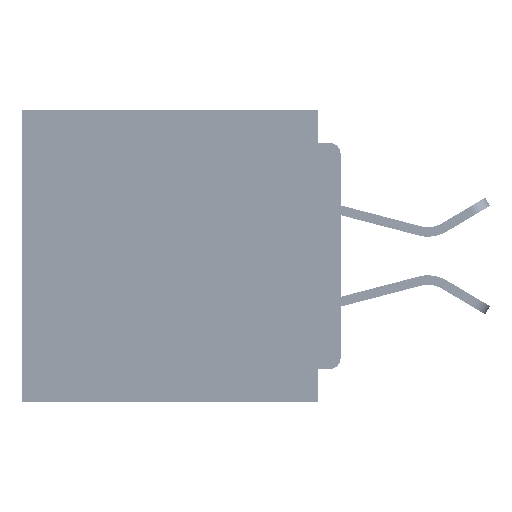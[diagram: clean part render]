
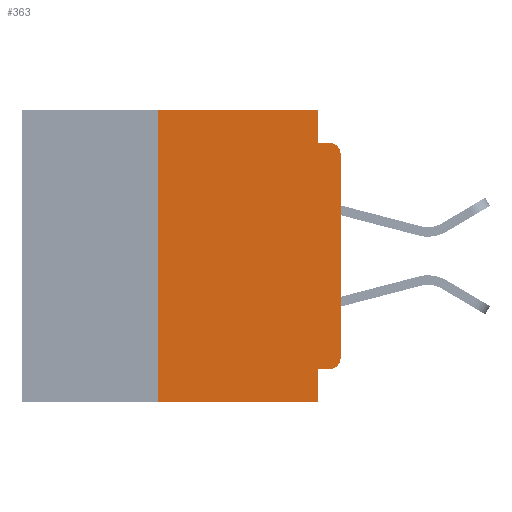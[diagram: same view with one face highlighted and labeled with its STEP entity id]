
A CAD part, left-side view. The second image highlights one B-rep face of the part: STEP entity #363.
In plain terms, the highlighted planar face has unit normal (-1, 0, 0).
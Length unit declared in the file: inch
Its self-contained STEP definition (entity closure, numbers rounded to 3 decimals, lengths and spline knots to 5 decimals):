
#234 = CARTESIAN_POINT ( 'NONE',  ( 0., 0.031, -0.045 ) ) ;
#363 = ADVANCED_FACE ( 'NONE', ( #35734 ), #36285, .F. ) ;
#1789 = DIRECTION ( 'NONE',  ( 0., 0., -1. ) ) ;
#2065 = AXIS2_PLACEMENT_3D ( 'NONE', #30913, #5976, #35728 ) ;
#2545 = EDGE_CURVE ( 'NONE', #19469, #3942, #49190, .T. ) ;
#3942 = VERTEX_POINT ( 'NONE', #12374 ) ;
#4067 = CARTESIAN_POINT ( 'NONE',  ( 0., 0.437, 0. ) ) ;
#4330 = ORIENTED_EDGE ( 'NONE', *, *, #42523, .T. ) ;
#4727 = CARTESIAN_POINT ( 'NONE',  ( 0., 0.031, -0.4 ) ) ;
#5724 = LINE ( 'NONE', #27153, #24837 ) ;
#5976 = DIRECTION ( 'NONE',  ( 1., 0., 0. ) ) ;
#6121 = LINE ( 'NONE', #38951, #37306 ) ;
#6165 = VECTOR ( 'NONE', #39838, 39.37008 ) ;
#6410 = ORIENTED_EDGE ( 'NONE', *, *, #41505, .T. ) ;
#7679 = LINE ( 'NONE', #4067, #26753 ) ;
#9474 = CARTESIAN_POINT ( 'NONE',  ( 0., 0.015, -0.045 ) ) ;
#10599 = LINE ( 'NONE', #19923, #30962 ) ;
#10759 = ORIENTED_EDGE ( 'NONE', *, *, #28411, .F. ) ;
#11155 = DIRECTION ( 'NONE',  ( 0., 0., 1. ) ) ;
#11517 = ORIENTED_EDGE ( 'NONE', *, *, #39396, .T. ) ;
#11683 = CARTESIAN_POINT ( 'NONE',  ( 0., 0.25, -0.4 ) ) ;
#11711 = EDGE_LOOP ( 'NONE', ( #11517, #6410, #13420, #52088, #10759, #29850, #4330, #13935, #52042, #15812 ) ) ;
#11923 = CARTESIAN_POINT ( 'NONE',  ( 0., 0.25, -0.4 ) ) ;
#12323 = EDGE_CURVE ( 'NONE', #33633, #23144, #5724, .T. ) ;
#12374 = CARTESIAN_POINT ( 'NONE',  ( 0., 0.25, 0. ) ) ;
#12680 = VERTEX_POINT ( 'NONE', #37437 ) ;
#12895 = VERTEX_POINT ( 'NONE', #23193 ) ;
#13278 = CARTESIAN_POINT ( 'NONE',  ( 0., 0.031, -0.355 ) ) ;
#13420 = ORIENTED_EDGE ( 'NONE', *, *, #12323, .F. ) ;
#13935 = ORIENTED_EDGE ( 'NONE', *, *, #35144, .F. ) ;
#13942 = CIRCLE ( 'NONE', #32953, 0.015 ) ;
#14894 = DIRECTION ( 'NONE',  ( 0., -1., 0. ) ) ;
#15812 = ORIENTED_EDGE ( 'NONE', *, *, #35626, .T. ) ;
#16298 = CARTESIAN_POINT ( 'NONE',  ( 0., 0., 0. ) ) ;
#16793 = VECTOR ( 'NONE', #11155, 39.37008 ) ;
#17746 = CARTESIAN_POINT ( 'NONE',  ( 0., 0.015, -0.34 ) ) ;
#18173 = EDGE_CURVE ( 'NONE', #12680, #33633, #27457, .T. ) ;
#18257 = LINE ( 'NONE', #35788, #6165 ) ;
#19469 = VERTEX_POINT ( 'NONE', #11923 ) ;
#19923 = CARTESIAN_POINT ( 'NONE',  ( 0., 0., -0.355 ) ) ;
#20084 = VERTEX_POINT ( 'NONE', #4727 ) ;
#20437 = VECTOR ( 'NONE', #48788, 39.37008 ) ;
#21707 = LINE ( 'NONE', #16298, #20437 ) ;
#21852 = DIRECTION ( 'NONE',  ( 0., 0., -1. ) ) ;
#23144 = VERTEX_POINT ( 'NONE', #9474 ) ;
#23193 = CARTESIAN_POINT ( 'NONE',  ( 0., 0., -0.06 ) ) ;
#23903 = CIRCLE ( 'NONE', #32817, 0.015 ) ;
#24019 = DIRECTION ( 'NONE',  ( 0., 1., 0. ) ) ;
#24179 = VERTEX_POINT ( 'NONE', #24302 ) ;
#24302 = CARTESIAN_POINT ( 'NONE',  ( 0., 0.015, -0.355 ) ) ;
#24837 = VECTOR ( 'NONE', #14894, 39.37008 ) ;
#24910 = VECTOR ( 'NONE', #43982, 39.37008 ) ;
#25299 = VERTEX_POINT ( 'NONE', #13278 ) ;
#26234 = DIRECTION ( 'NONE',  ( -1., 0., 0. ) ) ;
#26714 = DIRECTION ( 'NONE',  ( 0., 0., -1. ) ) ;
#26753 = VECTOR ( 'NONE', #48884, 39.37008 ) ;
#27153 = CARTESIAN_POINT ( 'NONE',  ( 0., 0., -0.045 ) ) ;
#27457 = LINE ( 'NONE', #27649, #24910 ) ;
#27649 = CARTESIAN_POINT ( 'NONE',  ( 0., 0.031, 0. ) ) ;
#28411 = EDGE_CURVE ( 'NONE', #3942, #12680, #7679, .T. ) ;
#29850 = ORIENTED_EDGE ( 'NONE', *, *, #2545, .F. ) ;
#30913 = CARTESIAN_POINT ( 'NONE',  ( 0., 0.437, 0. ) ) ;
#30962 = VECTOR ( 'NONE', #24019, 39.37008 ) ;
#32817 = AXIS2_PLACEMENT_3D ( 'NONE', #17746, #46175, #21852 ) ;
#32953 = AXIS2_PLACEMENT_3D ( 'NONE', #50543, #26234, #1789 ) ;
#33633 = VERTEX_POINT ( 'NONE', #234 ) ;
#35144 = EDGE_CURVE ( 'NONE', #25299, #20084, #6121, .T. ) ;
#35626 = EDGE_CURVE ( 'NONE', #24179, #52208, #23903, .T. ) ;
#35728 = DIRECTION ( 'NONE',  ( 0., 0., -1. ) ) ;
#35734 = FACE_OUTER_BOUND ( 'NONE', #11711, .T. ) ;
#35788 = CARTESIAN_POINT ( 'NONE',  ( 0., 0.437, -0.4 ) ) ;
#36285 = PLANE ( 'NONE',  #2065 ) ;
#37306 = VECTOR ( 'NONE', #26714, 39.37008 ) ;
#37437 = CARTESIAN_POINT ( 'NONE',  ( 0., 0.031, 0. ) ) ;
#38951 = CARTESIAN_POINT ( 'NONE',  ( 0., 0.031, -0.4 ) ) ;
#39396 = EDGE_CURVE ( 'NONE', #52208, #12895, #21707, .T. ) ;
#39838 = DIRECTION ( 'NONE',  ( 0., -1., 0. ) ) ;
#41505 = EDGE_CURVE ( 'NONE', #12895, #23144, #13942, .T. ) ;
#42523 = EDGE_CURVE ( 'NONE', #19469, #20084, #18257, .T. ) ;
#43123 = CARTESIAN_POINT ( 'NONE',  ( 0., 0., -0.34 ) ) ;
#43982 = DIRECTION ( 'NONE',  ( 0., 0., -1. ) ) ;
#46175 = DIRECTION ( 'NONE',  ( -1., 0., 0. ) ) ;
#46402 = EDGE_CURVE ( 'NONE', #24179, #25299, #10599, .T. ) ;
#48788 = DIRECTION ( 'NONE',  ( 0., 0., 1. ) ) ;
#48884 = DIRECTION ( 'NONE',  ( 0., -1., 0. ) ) ;
#49190 = LINE ( 'NONE', #11683, #16793 ) ;
#50543 = CARTESIAN_POINT ( 'NONE',  ( 0., 0.015, -0.06 ) ) ;
#52042 = ORIENTED_EDGE ( 'NONE', *, *, #46402, .F. ) ;
#52088 = ORIENTED_EDGE ( 'NONE', *, *, #18173, .F. ) ;
#52208 = VERTEX_POINT ( 'NONE', #43123 ) ;
